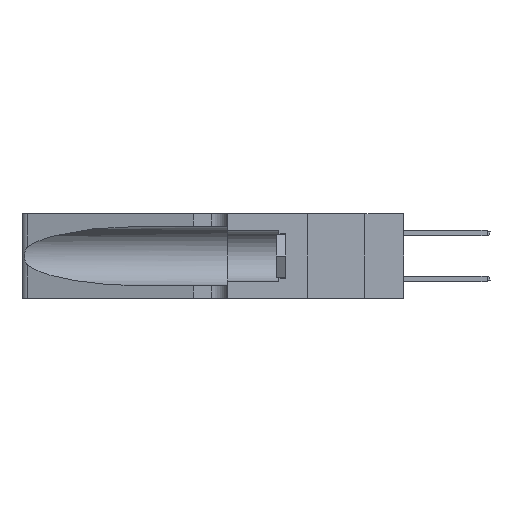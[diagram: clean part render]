
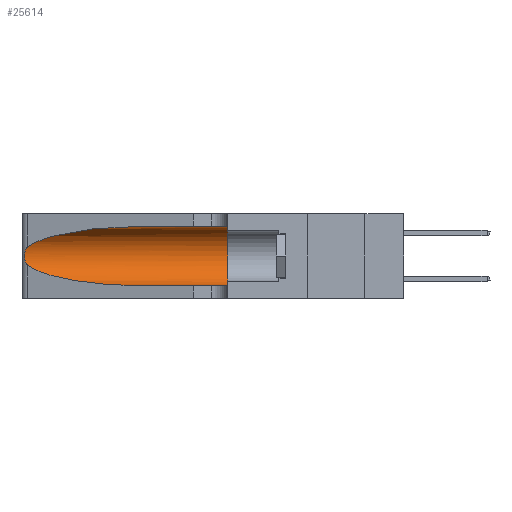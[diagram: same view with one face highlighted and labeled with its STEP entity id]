
A CAD part, left-side view. The second image highlights one B-rep face of the part: STEP entity #25614.
In plain terms, the highlighted cylindrical face has radius 3.308 mm (diameter 6.617 mm), a partial arc.
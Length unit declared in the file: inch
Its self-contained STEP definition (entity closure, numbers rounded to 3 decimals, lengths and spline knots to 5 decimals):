
#105 = CARTESIAN_POINT ( 'NONE',  ( 0.1305, 0.35, 0.31525 ) ) ;
#891 = ORIENTED_EDGE ( 'NONE', *, *, #21558, .T. ) ;
#1144 = ORIENTED_EDGE ( 'NONE', *, *, #4849, .F. ) ;
#1711 = VECTOR ( 'NONE', #14021, 39.37008 ) ;
#1944 = CARTESIAN_POINT ( 'NONE',  ( 0.26018, 1.23835, 0.19895 ) ) ;
#3980 = CARTESIAN_POINT ( 'NONE',  ( 0.1305, 1.61858, 0.31525 ) ) ;
#4009 = AXIS2_PLACEMENT_3D ( 'NONE', #8787, #23588, #10911 ) ;
#4135 = CARTESIAN_POINT ( 'NONE',  ( 0.26075, 1.23896, 0.178 ) ) ;
#4556 = CARTESIAN_POINT ( 'NONE',  ( 0.25487, 1.22718, 0.14631 ) ) ;
#4849 = EDGE_CURVE ( 'NONE', #20553, #5631, #14853, .T. ) ;
#5249 = EDGE_CURVE ( 'NONE', #21316, #14814, #15151, .T. ) ;
#5369 = CARTESIAN_POINT ( 'NONE',  ( 0.25487, 1.22718, 0.22369 ) ) ;
#5631 = VERTEX_POINT ( 'NONE', #20445 ) ;
#6079 = CARTESIAN_POINT ( 'NONE',  ( 0.25487, 1.22718, 0.22369 ) ) ;
#6252 = CARTESIAN_POINT ( 'NONE',  ( 0.25856, 1.23593, 0.16098 ) ) ;
#8098 = CARTESIAN_POINT ( 'NONE',  ( 0.1305, 0.72297, 0.31525 ) ) ;
#8162 =( BOUNDED_CURVE ( )  B_SPLINE_CURVE ( 3, ( #26414, #11688, #18091, #5369 ),
 .UNSPECIFIED., .F., .T. ) 
 B_SPLINE_CURVE_WITH_KNOTS ( ( 4, 4 ),
 ( 1.5708, 2.84003 ),
 .UNSPECIFIED. ) 
 CURVE ( )  GEOMETRIC_REPRESENTATION_ITEM ( )  RATIONAL_B_SPLINE_CURVE ( ( 1., 0.87, 0.87, 1. ) ) 
 REPRESENTATION_ITEM ( '' )  );
#8405 = CARTESIAN_POINT ( 'NONE',  ( 0.25639, 1.23186, 0.15144 ) ) ;
#8787 = CARTESIAN_POINT ( 'NONE',  ( 0.1305, 0.35, 0.185 ) ) ;
#10452 = CARTESIAN_POINT ( 'NONE',  ( 0.25555, 1.22994, 0.2215 ) ) ;
#10529 = CARTESIAN_POINT ( 'NONE',  ( 0.25487, 1.22718, 0.14631 ) ) ;
#10545 = CARTESIAN_POINT ( 'NONE',  ( 0.25487, 1.22718, 0.14631 ) ) ;
#10911 = DIRECTION ( 'NONE',  ( 0., 0., 1. ) ) ;
#11407 = FACE_OUTER_BOUND ( 'NONE', #11534, .T. ) ;
#11534 = EDGE_LOOP ( 'NONE', ( #891, #17462, #20823, #27304, #1144, #15535 ) ) ;
#11688 = CARTESIAN_POINT ( 'NONE',  ( 0.18966, 0.96281, 0.31525 ) ) ;
#11860 = VECTOR ( 'NONE', #14581, 39.37008 ) ;
#11886 = CARTESIAN_POINT ( 'NONE',  ( 0.1305, 1.61858, 0.05475 ) ) ;
#12595 = CARTESIAN_POINT ( 'NONE',  ( 0.25639, 1.23184, 0.21858 ) ) ;
#12669 = CARTESIAN_POINT ( 'NONE',  ( 0.1305, 0.72297, 0.05475 ) ) ;
#13022 = VERTEX_POINT ( 'NONE', #16485 ) ;
#13472 = DIRECTION ( 'NONE',  ( 0., -1., 0. ) ) ;
#13749 = LINE ( 'NONE', #11886, #1711 ) ;
#14021 = DIRECTION ( 'NONE',  ( 0., -1., 0. ) ) ;
#14581 = DIRECTION ( 'NONE',  ( 0., -1., 0. ) ) ;
#14730 = CARTESIAN_POINT ( 'NONE',  ( 0.25854, 1.2359, 0.20912 ) ) ;
#14814 = VERTEX_POINT ( 'NONE', #22374 ) ;
#14853 = CIRCLE ( 'NONE', #4009, 0.13025 ) ;
#15151 =( BOUNDED_CURVE ( )  B_SPLINE_CURVE ( 3, ( #10529, #27296, #16846, #12669 ),
 .UNSPECIFIED., .F., .F. ) 
 B_SPLINE_CURVE_WITH_KNOTS ( ( 4, 4 ),
 ( 3.44316, 4.71239 ),
 .UNSPECIFIED. ) 
 CURVE ( )  GEOMETRIC_REPRESENTATION_ITEM ( )  RATIONAL_B_SPLINE_CURVE ( ( 1., 0.87, 0.87, 1. ) ) 
 REPRESENTATION_ITEM ( '' )  );
#15535 = ORIENTED_EDGE ( 'NONE', *, *, #17803, .F. ) ;
#16485 = CARTESIAN_POINT ( 'NONE',  ( 0.25487, 1.22718, 0.22369 ) ) ;
#16846 = CARTESIAN_POINT ( 'NONE',  ( 0.18966, 0.96281, 0.05475 ) ) ;
#16856 = CARTESIAN_POINT ( 'NONE',  ( 0.26075, 1.23896, 0.19203 ) ) ;
#17030 = VERTEX_POINT ( 'NONE', #8098 ) ;
#17462 = ORIENTED_EDGE ( 'NONE', *, *, #18478, .T. ) ;
#17803 = EDGE_CURVE ( 'NONE', #17030, #20553, #18849, .T. ) ;
#18040 = B_SPLINE_CURVE_WITH_KNOTS ( 'NONE', 3,
 ( #6079, #10452, #12595, #27309, #14730, #1944, #16856, #4135, #19009, #6252, #21137, #8405, #23226, #10545 ),
 .UNSPECIFIED., .F., .F.,
 ( 4, 2, 2, 2, 2, 2, 4 ),
 ( 0., 0.00027, 0.00053, 0.00107, 0.0016, 0.00187, 0.00214 ),
 .UNSPECIFIED. ) ;
#18091 = CARTESIAN_POINT ( 'NONE',  ( 0.2373, 1.15595, 0.28018 ) ) ;
#18478 = EDGE_CURVE ( 'NONE', #13022, #21316, #18040, .T. ) ;
#18849 = LINE ( 'NONE', #3980, #11860 ) ;
#19009 = CARTESIAN_POINT ( 'NONE',  ( 0.26017, 1.23833, 0.17102 ) ) ;
#19560 = EDGE_CURVE ( 'NONE', #14814, #5631, #13749, .T. ) ;
#20445 = CARTESIAN_POINT ( 'NONE',  ( 0.1305, 0.35, 0.05475 ) ) ;
#20553 = VERTEX_POINT ( 'NONE', #105 ) ;
#20823 = ORIENTED_EDGE ( 'NONE', *, *, #5249, .T. ) ;
#21137 = CARTESIAN_POINT ( 'NONE',  ( 0.25789, 1.23486, 0.15765 ) ) ;
#21316 = VERTEX_POINT ( 'NONE', #4556 ) ;
#21558 = EDGE_CURVE ( 'NONE', #17030, #13022, #8162, .T. ) ;
#21935 = AXIS2_PLACEMENT_3D ( 'NONE', #23980, #13472, #26053 ) ;
#22374 = CARTESIAN_POINT ( 'NONE',  ( 0.1305, 0.72297, 0.05475 ) ) ;
#23226 = CARTESIAN_POINT ( 'NONE',  ( 0.25555, 1.22993, 0.14849 ) ) ;
#23588 = DIRECTION ( 'NONE',  ( 0., 1., 0. ) ) ;
#23980 = CARTESIAN_POINT ( 'NONE',  ( 0.1305, 1.61858, 0.185 ) ) ;
#25614 = ADVANCED_FACE ( 'NONE', ( #11407 ), #26889, .F. ) ;
#26053 = DIRECTION ( 'NONE',  ( 0., 0., -1. ) ) ;
#26414 = CARTESIAN_POINT ( 'NONE',  ( 0.1305, 0.72297, 0.31525 ) ) ;
#26889 = CYLINDRICAL_SURFACE ( 'NONE', #21935, 0.13025 ) ;
#27296 = CARTESIAN_POINT ( 'NONE',  ( 0.2373, 1.15595, 0.08982 ) ) ;
#27304 = ORIENTED_EDGE ( 'NONE', *, *, #19560, .T. ) ;
#27309 = CARTESIAN_POINT ( 'NONE',  ( 0.25787, 1.23484, 0.2124 ) ) ;
